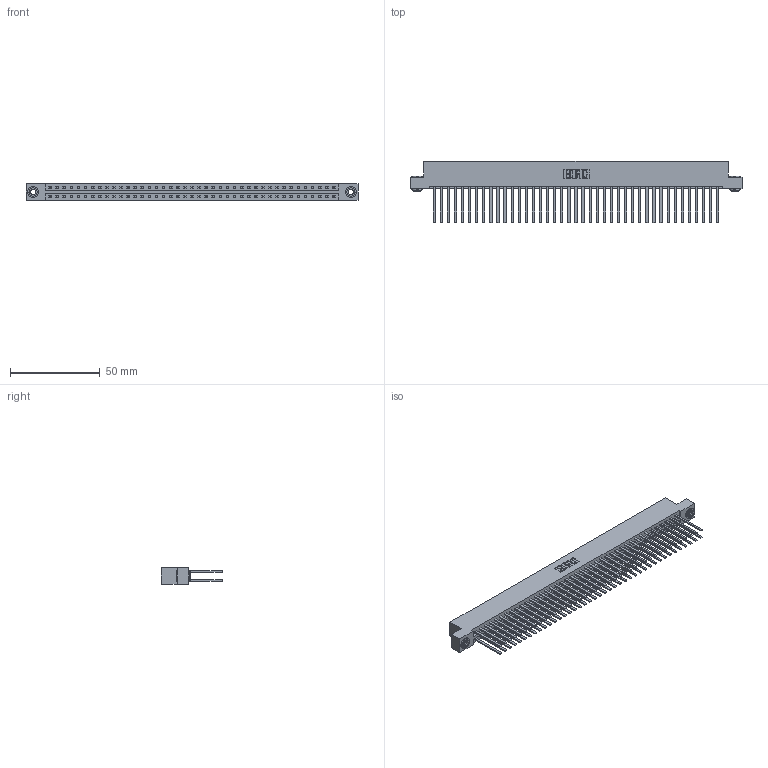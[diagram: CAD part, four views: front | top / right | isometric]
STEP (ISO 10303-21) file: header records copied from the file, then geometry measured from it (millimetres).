
FILE_DESCRIPTION (( 'STEP AP203' ), '1' );
FILE_NAME ('387-082-544-203.STEP', '2019-10-22T23:57:37', ( '' ), ( '' ), 'SwSTEP 2.0', 'SolidWorks 2016', '' );
FILE_SCHEMA (( 'CONFIG_CONTROL_DESIGN' ));
Length unit declared in the file: inch
Products named in the file (4): 345-250-002_345-250-002-102; 345-292-001_345-293-144; 387-082-544-203; 337 Part_Flush Mounting Lugs - 0.156 Dia-TH
Assembly tree (85 placements, depth 2):
  387-082-544-203
    337 Part_Flush Mounting Lugs - 0.156 Dia-TH
    345-292-001_345-293-144  x82
    345-250-002_345-250-002-102  x2
Bounding box: 185.47 x 34.3 x 9.4 mm (x, y, z)
Volume: 20702 mm3; surface area: 27373.4 mm2
Topology: 85 solids, 85 shells, 4088 faces, 12113 edges, 7962 vertices
Faces by surface type: plane 2868, cylinder 1212, cone 8
Entity records: 32384 total; most frequent: CARTESIAN_POINT 5429, ORIENTED_EDGE 5358, DIRECTION 4649, EDGE_CURVE 2679, VECTOR 2531, LINE 2531, VERTEX_POINT 1782, AXIS2_PLACEMENT_3D 1059
